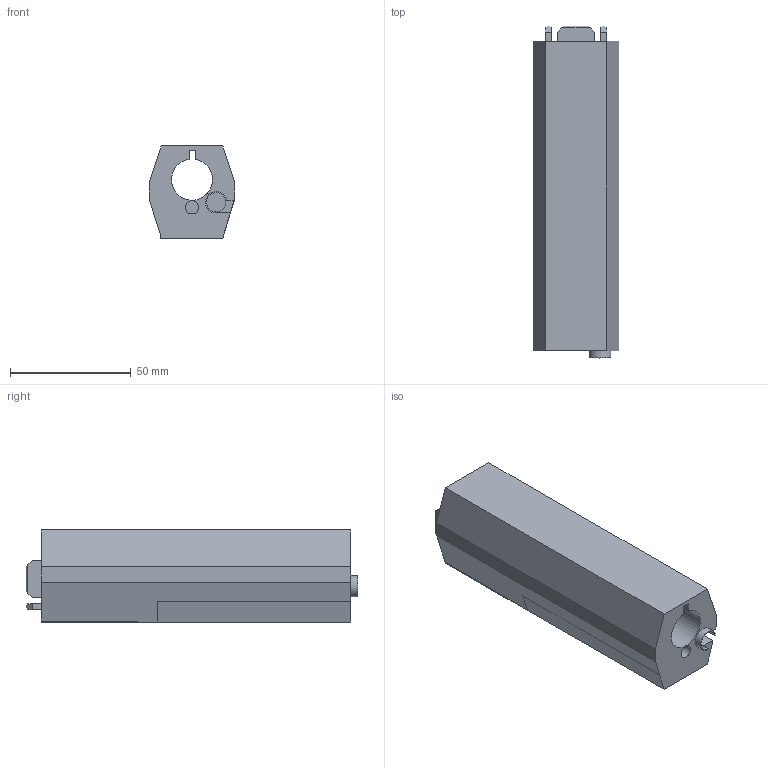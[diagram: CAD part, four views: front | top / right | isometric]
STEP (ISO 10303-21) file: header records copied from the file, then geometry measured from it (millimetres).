
FILE_DESCRIPTION(/* description */ (''),/* implementation_level */ '2;1');
FILE_NAME(/* name */ '79db9c0d-4e9e-4b57-b568-bffef17fa9d4.stp',/* time_stamp */ '2019-11-26T06:10:40+00:00',/* author */ (''),/* organization */ (''),/* preprocessor_version */ 'ST-DEVELOPER v18',/* originating_system */ 'Autodesk Translation Framework v8.12.0.6',/* authorisation */ '');
FILE_SCHEMA (('AUTOMOTIVE_DESIGN { 1 0 10303 214 3 1 1 }'));
Length unit declared in the file: inch
Products named in the file (1): Heritage Rough Rider - Fore End Base
Bounding box: 35.56 x 137.37 x 38.1 mm (x, y, z)
Volume: 117177 mm3; surface area: 29310 mm2
Topology: 1 solids, 1 shells, 63 faces, 169 edges, 113 vertices
Faces by surface type: plane 56, cylinder 7
Full cylindrical faces by diameter (mm): 3 x1, 4.8 x1, 5.5 x1
Entity records: 2019 total; most frequent: CARTESIAN_POINT 380, ORIENTED_EDGE 338, DIRECTION 310, EDGE_CURVE 169, LINE 152, VECTOR 152, VERTEX_POINT 113, AXIS2_PLACEMENT_3D 79
